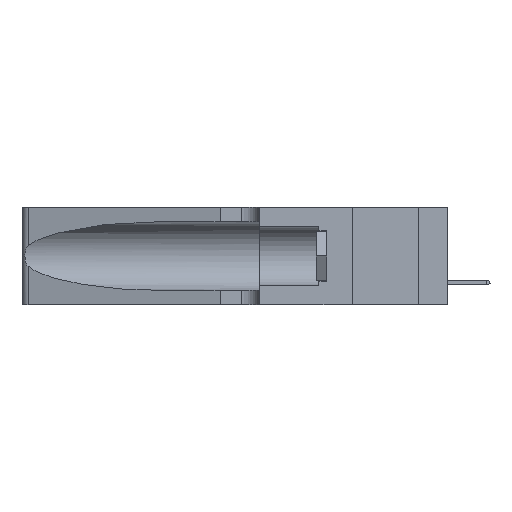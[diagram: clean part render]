
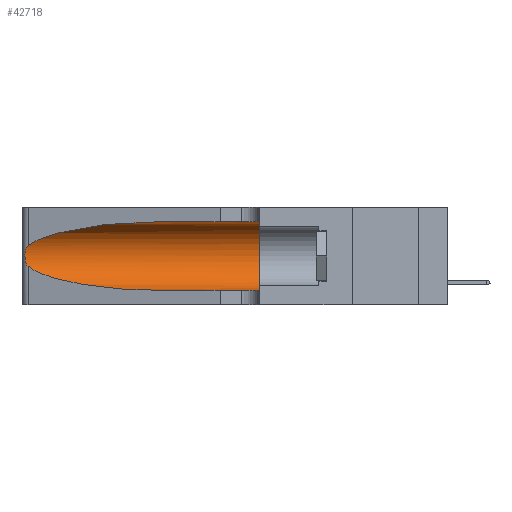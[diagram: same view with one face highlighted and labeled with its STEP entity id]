
A CAD part, left-side view. The second image highlights one B-rep face of the part: STEP entity #42718.
In plain terms, the highlighted cylindrical face has radius 3.308 mm (diameter 6.617 mm), a partial arc.
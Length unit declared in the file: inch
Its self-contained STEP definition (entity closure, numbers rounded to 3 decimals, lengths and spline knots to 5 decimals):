
#62 = VERTEX_POINT ( 'NONE', #5023 ) ;
#2298 = CARTESIAN_POINT ( 'NONE',  ( 0.1305, 0.72297, 0.05475 ) ) ;
#2581 = EDGE_CURVE ( 'NONE', #23694, #62, #12387, .T. ) ;
#2636 = FACE_OUTER_BOUND ( 'NONE', #38735, .T. ) ;
#2889 = CARTESIAN_POINT ( 'NONE',  ( 0.1305, 0.72297, 0.31525 ) ) ;
#3137 = CARTESIAN_POINT ( 'NONE',  ( 0.25555, 1.22993, 0.14849 ) ) ;
#5023 = CARTESIAN_POINT ( 'NONE',  ( 0.1305, 0.72297, 0.05475 ) ) ;
#5375 = LINE ( 'NONE', #11468, #32426 ) ;
#5955 = ORIENTED_EDGE ( 'NONE', *, *, #35882, .F. ) ;
#6818 = CARTESIAN_POINT ( 'NONE',  ( 0.25487, 1.22718, 0.14631 ) ) ;
#6964 = AXIS2_PLACEMENT_3D ( 'NONE', #39073, #9796, #17852 ) ;
#7555 = DIRECTION ( 'NONE',  ( 0., 1., 0. ) ) ;
#8512 = CARTESIAN_POINT ( 'NONE',  ( 0.25487, 1.22718, 0.14631 ) ) ;
#8897 = DIRECTION ( 'NONE',  ( 0., -1., 0. ) ) ;
#9058 = CARTESIAN_POINT ( 'NONE',  ( 0.1305, 0.35, 0.05475 ) ) ;
#9651 = CARTESIAN_POINT ( 'NONE',  ( 0.2373, 1.15595, 0.08982 ) ) ;
#9745 = B_SPLINE_CURVE_WITH_KNOTS ( 'NONE', 3,
 ( #39831, #32562, #18111, #40578, #29657, #11301, #15167, #33605, #41663, #12740, #37180, #31427, #3137, #6818 ),
 .UNSPECIFIED., .F., .F.,
 ( 4, 2, 2, 2, 2, 2, 4 ),
 ( 0., 0.00027, 0.00053, 0.00107, 0.0016, 0.00187, 0.00214 ),
 .UNSPECIFIED. ) ;
#9796 = DIRECTION ( 'NONE',  ( 0., -1., 0. ) ) ;
#10082 = CARTESIAN_POINT ( 'NONE',  ( 0.18966, 0.96281, 0.31525 ) ) ;
#10480 = EDGE_CURVE ( 'NONE', #31634, #36090, #37455, .T. ) ;
#10730 = AXIS2_PLACEMENT_3D ( 'NONE', #18456, #7555, #43901 ) ;
#11301 = CARTESIAN_POINT ( 'NONE',  ( 0.26018, 1.23835, 0.19895 ) ) ;
#11468 = CARTESIAN_POINT ( 'NONE',  ( 0.1305, 1.61858, 0.31525 ) ) ;
#11895 = EDGE_CURVE ( 'NONE', #36090, #23694, #9745, .T. ) ;
#12283 = LINE ( 'NONE', #31110, #25576 ) ;
#12387 =( BOUNDED_CURVE ( )  B_SPLINE_CURVE ( 3, ( #34051, #9651, #42292, #2298 ),
 .UNSPECIFIED., .F., .T. ) 
 B_SPLINE_CURVE_WITH_KNOTS ( ( 4, 4 ),
 ( 3.44316, 4.71239 ),
 .UNSPECIFIED. ) 
 CURVE ( )  GEOMETRIC_REPRESENTATION_ITEM ( )  RATIONAL_B_SPLINE_CURVE ( ( 1., 0.87, 0.87, 1. ) ) 
 REPRESENTATION_ITEM ( '' )  );
#12629 = DIRECTION ( 'NONE',  ( 0., -1., 0. ) ) ;
#12740 = CARTESIAN_POINT ( 'NONE',  ( 0.25856, 1.23593, 0.16098 ) ) ;
#15167 = CARTESIAN_POINT ( 'NONE',  ( 0.26075, 1.23896, 0.19203 ) ) ;
#16171 = EDGE_CURVE ( 'NONE', #62, #26221, #12283, .T. ) ;
#17852 = DIRECTION ( 'NONE',  ( 0., 0., -1. ) ) ;
#18034 = ORIENTED_EDGE ( 'NONE', *, *, #37634, .F. ) ;
#18111 = CARTESIAN_POINT ( 'NONE',  ( 0.25639, 1.23184, 0.21858 ) ) ;
#18456 = CARTESIAN_POINT ( 'NONE',  ( 0.1305, 0.35, 0.185 ) ) ;
#18731 = CIRCLE ( 'NONE', #10730, 0.13025 ) ;
#21209 = CARTESIAN_POINT ( 'NONE',  ( 0.1305, 0.72297, 0.31525 ) ) ;
#23694 = VERTEX_POINT ( 'NONE', #8512 ) ;
#25576 = VECTOR ( 'NONE', #12629, 39.37008 ) ;
#25790 = ORIENTED_EDGE ( 'NONE', *, *, #16171, .T. ) ;
#26144 = ORIENTED_EDGE ( 'NONE', *, *, #2581, .T. ) ;
#26221 = VERTEX_POINT ( 'NONE', #9058 ) ;
#26562 = ORIENTED_EDGE ( 'NONE', *, *, #11895, .T. ) ;
#29657 = CARTESIAN_POINT ( 'NONE',  ( 0.25854, 1.2359, 0.20912 ) ) ;
#30935 = ORIENTED_EDGE ( 'NONE', *, *, #10480, .T. ) ;
#31110 = CARTESIAN_POINT ( 'NONE',  ( 0.1305, 1.61858, 0.05475 ) ) ;
#31427 = CARTESIAN_POINT ( 'NONE',  ( 0.25639, 1.23186, 0.15144 ) ) ;
#31634 = VERTEX_POINT ( 'NONE', #2889 ) ;
#32426 = VECTOR ( 'NONE', #8897, 39.37008 ) ;
#32562 = CARTESIAN_POINT ( 'NONE',  ( 0.25555, 1.22994, 0.2215 ) ) ;
#33437 = VERTEX_POINT ( 'NONE', #33630 ) ;
#33605 = CARTESIAN_POINT ( 'NONE',  ( 0.26075, 1.23896, 0.178 ) ) ;
#33630 = CARTESIAN_POINT ( 'NONE',  ( 0.1305, 0.35, 0.31525 ) ) ;
#34051 = CARTESIAN_POINT ( 'NONE',  ( 0.25487, 1.22718, 0.14631 ) ) ;
#35882 = EDGE_CURVE ( 'NONE', #33437, #26221, #18731, .T. ) ;
#36090 = VERTEX_POINT ( 'NONE', #39721 ) ;
#37180 = CARTESIAN_POINT ( 'NONE',  ( 0.25789, 1.23486, 0.15765 ) ) ;
#37455 =( BOUNDED_CURVE ( )  B_SPLINE_CURVE ( 3, ( #21209, #10082, #37915, #46767 ),
 .UNSPECIFIED., .F., .F. ) 
 B_SPLINE_CURVE_WITH_KNOTS ( ( 4, 4 ),
 ( 1.5708, 2.84003 ),
 .UNSPECIFIED. ) 
 CURVE ( )  GEOMETRIC_REPRESENTATION_ITEM ( )  RATIONAL_B_SPLINE_CURVE ( ( 1., 0.87, 0.87, 1. ) ) 
 REPRESENTATION_ITEM ( '' )  );
#37634 = EDGE_CURVE ( 'NONE', #31634, #33437, #5375, .T. ) ;
#37915 = CARTESIAN_POINT ( 'NONE',  ( 0.2373, 1.15595, 0.28018 ) ) ;
#38735 = EDGE_LOOP ( 'NONE', ( #30935, #26562, #26144, #25790, #5955, #18034 ) ) ;
#39073 = CARTESIAN_POINT ( 'NONE',  ( 0.1305, 1.61858, 0.185 ) ) ;
#39721 = CARTESIAN_POINT ( 'NONE',  ( 0.25487, 1.22718, 0.22369 ) ) ;
#39831 = CARTESIAN_POINT ( 'NONE',  ( 0.25487, 1.22718, 0.22369 ) ) ;
#40578 = CARTESIAN_POINT ( 'NONE',  ( 0.25787, 1.23484, 0.2124 ) ) ;
#41663 = CARTESIAN_POINT ( 'NONE',  ( 0.26017, 1.23833, 0.17102 ) ) ;
#42292 = CARTESIAN_POINT ( 'NONE',  ( 0.18966, 0.96281, 0.05475 ) ) ;
#42718 = ADVANCED_FACE ( 'NONE', ( #2636 ), #47516, .F. ) ;
#43901 = DIRECTION ( 'NONE',  ( 0., 0., 1. ) ) ;
#46767 = CARTESIAN_POINT ( 'NONE',  ( 0.25487, 1.22718, 0.22369 ) ) ;
#47516 = CYLINDRICAL_SURFACE ( 'NONE', #6964, 0.13025 ) ;
